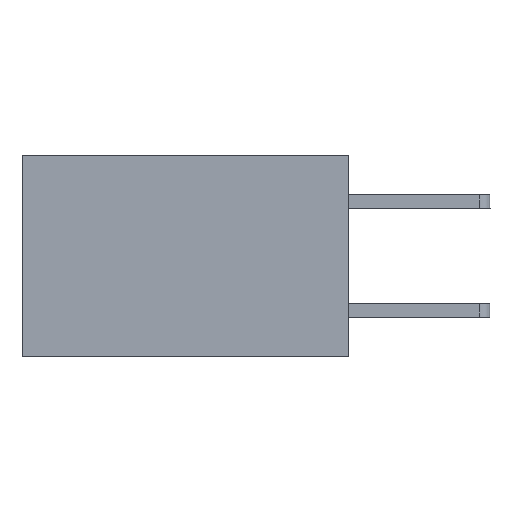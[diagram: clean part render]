
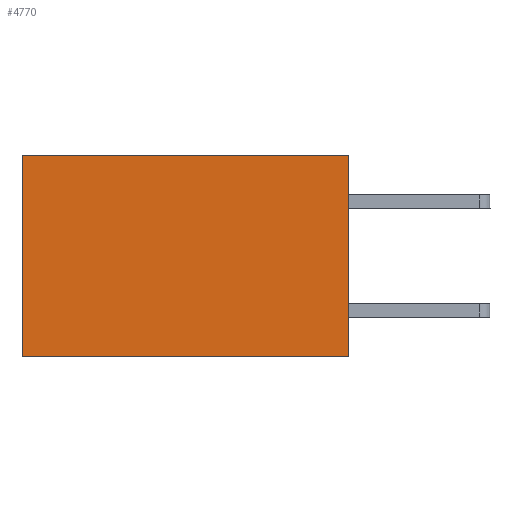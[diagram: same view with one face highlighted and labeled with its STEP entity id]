
A CAD part, left-side view. The second image highlights one B-rep face of the part: STEP entity #4770.
In plain terms, the highlighted planar face has unit normal (-1, 0, 0).
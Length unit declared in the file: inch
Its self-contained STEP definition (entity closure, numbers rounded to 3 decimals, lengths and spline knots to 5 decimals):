
#47 = ORIENTED_EDGE ( 'NONE', *, *, #3249, .T. ) ;
#84 = CARTESIAN_POINT ( 'NONE',  ( 0.2615, 0.6, -0.37 ) ) ;
#500 = VERTEX_POINT ( 'NONE', #6161 ) ;
#532 = DIRECTION ( 'NONE',  ( 0., 1., 0. ) ) ;
#563 = LINE ( 'NONE', #700, #7244 ) ;
#656 = PLANE ( 'NONE',  #6078 ) ;
#700 = CARTESIAN_POINT ( 'NONE',  ( 0.2615, 0., 0. ) ) ;
#717 = ORIENTED_EDGE ( 'NONE', *, *, #1726, .F. ) ;
#1726 = EDGE_CURVE ( 'NONE', #500, #4448, #3871, .T. ) ;
#1861 = CARTESIAN_POINT ( 'NONE',  ( 0.2615, 0.6, 0. ) ) ;
#2018 = CARTESIAN_POINT ( 'NONE',  ( 0.2615, 0., -0.37 ) ) ;
#3084 = CARTESIAN_POINT ( 'NONE',  ( 0.2615, 0., 0. ) ) ;
#3128 = ORIENTED_EDGE ( 'NONE', *, *, #5940, .T. ) ;
#3249 = EDGE_CURVE ( 'NONE', #6917, #4448, #5510, .T. ) ;
#3344 = CARTESIAN_POINT ( 'NONE',  ( 0.2615, 0., -0.37 ) ) ;
#3492 = EDGE_CURVE ( 'NONE', #4624, #500, #3907, .T. ) ;
#3871 = LINE ( 'NONE', #5961, #5752 ) ;
#3907 = LINE ( 'NONE', #2018, #5050 ) ;
#3999 = DIRECTION ( 'NONE',  ( 0., 1., 0. ) ) ;
#4448 = VERTEX_POINT ( 'NONE', #84 ) ;
#4624 = VERTEX_POINT ( 'NONE', #3084 ) ;
#4698 = DIRECTION ( 'NONE',  ( 0., 0., -1. ) ) ;
#4770 = ADVANCED_FACE ( 'NONE', ( #7371 ), #656, .F. ) ;
#5050 = VECTOR ( 'NONE', #4698, 39.37008 ) ;
#5510 = LINE ( 'NONE', #7557, #5627 ) ;
#5627 = VECTOR ( 'NONE', #6137, 39.37008 ) ;
#5752 = VECTOR ( 'NONE', #532, 39.37008 ) ;
#5912 = DIRECTION ( 'NONE',  ( 0., 0., -1. ) ) ;
#5940 = EDGE_CURVE ( 'NONE', #4624, #6917, #563, .T. ) ;
#5961 = CARTESIAN_POINT ( 'NONE',  ( 0.2615, 0., -0.37 ) ) ;
#6078 = AXIS2_PLACEMENT_3D ( 'NONE', #3344, #8062, #5912 ) ;
#6137 = DIRECTION ( 'NONE',  ( 0., 0., -1. ) ) ;
#6161 = CARTESIAN_POINT ( 'NONE',  ( 0.2615, 0., -0.37 ) ) ;
#6917 = VERTEX_POINT ( 'NONE', #1861 ) ;
#6927 = ORIENTED_EDGE ( 'NONE', *, *, #3492, .F. ) ;
#7244 = VECTOR ( 'NONE', #3999, 39.37008 ) ;
#7371 = FACE_OUTER_BOUND ( 'NONE', #8163, .T. ) ;
#7557 = CARTESIAN_POINT ( 'NONE',  ( 0.2615, 0.6, -0.37 ) ) ;
#8062 = DIRECTION ( 'NONE',  ( 1., 0., 0. ) ) ;
#8163 = EDGE_LOOP ( 'NONE', ( #47, #717, #6927, #3128 ) ) ;
